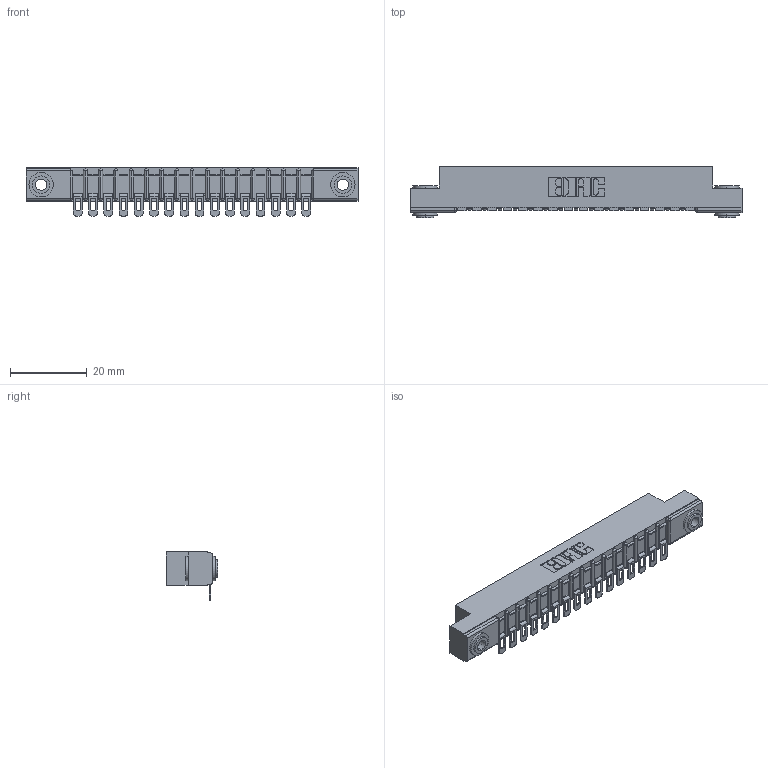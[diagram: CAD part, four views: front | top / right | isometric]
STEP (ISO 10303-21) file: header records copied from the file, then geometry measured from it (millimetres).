
FILE_DESCRIPTION (( 'STEP AP203' ), '1' );
FILE_NAME ('357-016-454-103.STEP', '2020-09-30T20:07:49', ( '' ), ( '' ), 'SwSTEP 2.0', 'SolidWorks 2020', '' );
FILE_SCHEMA (( 'CONFIG_CONTROL_DESIGN' ));
Length unit declared in the file: inch
Products named in the file (4): 307 Part_.156 Dia Mounting Holes; 357-016-454-103; 345-250-002_345-250-002-102; 307-290-002_554
Assembly tree (19 placements, depth 2):
  357-016-454-103
    307 Part_.156 Dia Mounting Holes
    307-290-002_554  x16
    345-250-002_345-250-002-102  x2
Bounding box: 86.41 x 13.36 x 12.52 mm (x, y, z)
Volume: 5708.6 mm3; surface area: 10359.1 mm2
Topology: 19 solids, 19 shells, 1483 faces, 4483 edges, 2938 vertices
Faces by surface type: plane 830, cylinder 611, sphere 34, cone 8
Entity records: 18952 total; most frequent: CARTESIAN_POINT 3171, ORIENTED_EDGE 3152, DIRECTION 3114, EDGE_CURVE 1576, VECTOR 1180, LINE 1180, VERTEX_POINT 1024, AXIS2_PLACEMENT_3D 967
